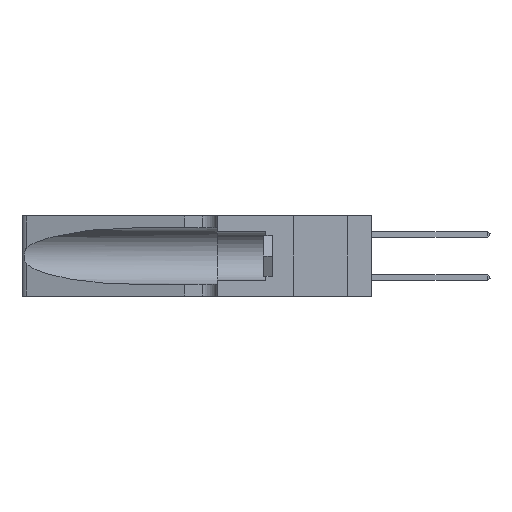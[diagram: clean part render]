
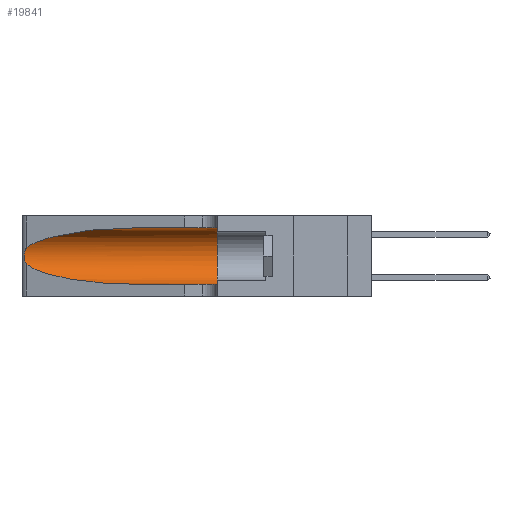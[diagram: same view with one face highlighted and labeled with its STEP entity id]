
A CAD part, left-side view. The second image highlights one B-rep face of the part: STEP entity #19841.
In plain terms, the highlighted cylindrical face has radius 3.308 mm (diameter 6.617 mm), a partial arc.
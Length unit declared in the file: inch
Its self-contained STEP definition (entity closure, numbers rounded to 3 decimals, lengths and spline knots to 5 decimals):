
#235 = CARTESIAN_POINT ( 'NONE',  ( 0.1305, 0.35, 0.185 ) ) ;
#570 = CARTESIAN_POINT ( 'NONE',  ( 0.25639, 1.23186, 0.15144 ) ) ;
#790 = CARTESIAN_POINT ( 'NONE',  ( 0.26017, 1.23833, 0.17102 ) ) ;
#1086 =( BOUNDED_CURVE ( )  B_SPLINE_CURVE ( 3, ( #15805, #12935, #13164, #20333 ),
 .UNSPECIFIED., .F., .F. ) 
 B_SPLINE_CURVE_WITH_KNOTS ( ( 4, 4 ),
 ( 1.5708, 2.84003 ),
 .UNSPECIFIED. ) 
 CURVE ( )  GEOMETRIC_REPRESENTATION_ITEM ( )  RATIONAL_B_SPLINE_CURVE ( ( 1., 0.87, 0.87, 1. ) ) 
 REPRESENTATION_ITEM ( '' )  );
#1731 = DIRECTION ( 'NONE',  ( 0., -1., 0. ) ) ;
#1955 = CARTESIAN_POINT ( 'NONE',  ( 0.1305, 1.61858, 0.31525 ) ) ;
#2019 = CIRCLE ( 'NONE', #22826, 0.13025 ) ;
#2462 = CARTESIAN_POINT ( 'NONE',  ( 0.2373, 1.15595, 0.08982 ) ) ;
#2648 = DIRECTION ( 'NONE',  ( 0., -1., 0. ) ) ;
#2991 = CARTESIAN_POINT ( 'NONE',  ( 0.25487, 1.22718, 0.14631 ) ) ;
#4802 = EDGE_CURVE ( 'NONE', #27854, #12663, #32027, .T. ) ;
#5497 = CARTESIAN_POINT ( 'NONE',  ( 0.25487, 1.22718, 0.22369 ) ) ;
#5634 = CARTESIAN_POINT ( 'NONE',  ( 0.25789, 1.23486, 0.15765 ) ) ;
#5841 = EDGE_CURVE ( 'NONE', #22460, #14654, #16721, .T. ) ;
#6043 = EDGE_CURVE ( 'NONE', #14654, #13248, #11455, .T. ) ;
#7438 = DIRECTION ( 'NONE',  ( 0., 0., 1. ) ) ;
#7979 = CARTESIAN_POINT ( 'NONE',  ( 0.26075, 1.23896, 0.178 ) ) ;
#7989 = ORIENTED_EDGE ( 'NONE', *, *, #20329, .F. ) ;
#8063 = CARTESIAN_POINT ( 'NONE',  ( 0.1305, 1.61858, 0.05475 ) ) ;
#8187 = CARTESIAN_POINT ( 'NONE',  ( 0.26075, 1.23896, 0.19203 ) ) ;
#10887 = CARTESIAN_POINT ( 'NONE',  ( 0.25787, 1.23484, 0.2124 ) ) ;
#11156 = ORIENTED_EDGE ( 'NONE', *, *, #4802, .F. ) ;
#11455 = LINE ( 'NONE', #8063, #18912 ) ;
#12663 = VERTEX_POINT ( 'NONE', #20535 ) ;
#12935 = CARTESIAN_POINT ( 'NONE',  ( 0.18966, 0.96281, 0.31525 ) ) ;
#13164 = CARTESIAN_POINT ( 'NONE',  ( 0.2373, 1.15595, 0.28018 ) ) ;
#13248 = VERTEX_POINT ( 'NONE', #27763 ) ;
#13956 = CYLINDRICAL_SURFACE ( 'NONE', #25717, 0.13025 ) ;
#14654 = VERTEX_POINT ( 'NONE', #27692 ) ;
#14758 = CARTESIAN_POINT ( 'NONE',  ( 0.1305, 0.72297, 0.05475 ) ) ;
#15805 = CARTESIAN_POINT ( 'NONE',  ( 0.1305, 0.72297, 0.31525 ) ) ;
#15926 = FACE_OUTER_BOUND ( 'NONE', #27767, .T. ) ;
#16721 =( BOUNDED_CURVE ( )  B_SPLINE_CURVE ( 3, ( #17593, #2462, #30049, #14758 ),
 .UNSPECIFIED., .F., .F. ) 
 B_SPLINE_CURVE_WITH_KNOTS ( ( 4, 4 ),
 ( 3.44316, 4.71239 ),
 .UNSPECIFIED. ) 
 CURVE ( )  GEOMETRIC_REPRESENTATION_ITEM ( )  RATIONAL_B_SPLINE_CURVE ( ( 1., 0.87, 0.87, 1. ) ) 
 REPRESENTATION_ITEM ( '' )  );
#17593 = CARTESIAN_POINT ( 'NONE',  ( 0.25487, 1.22718, 0.14631 ) ) ;
#17687 = VERTEX_POINT ( 'NONE', #5497 ) ;
#18127 = CARTESIAN_POINT ( 'NONE',  ( 0.25856, 1.23593, 0.16098 ) ) ;
#18912 = VECTOR ( 'NONE', #2648, 39.37008 ) ;
#19402 = DIRECTION ( 'NONE',  ( 0., -1., 0. ) ) ;
#19419 = VECTOR ( 'NONE', #1731, 39.37008 ) ;
#19627 = ORIENTED_EDGE ( 'NONE', *, *, #25099, .T. ) ;
#19841 = ADVANCED_FACE ( 'NONE', ( #15926 ), #13956, .F. ) ;
#20329 = EDGE_CURVE ( 'NONE', #12663, #13248, #2019, .T. ) ;
#20333 = CARTESIAN_POINT ( 'NONE',  ( 0.25487, 1.22718, 0.22369 ) ) ;
#20535 = CARTESIAN_POINT ( 'NONE',  ( 0.1305, 0.35, 0.31525 ) ) ;
#20575 = CARTESIAN_POINT ( 'NONE',  ( 0.25555, 1.22994, 0.2215 ) ) ;
#21088 = ORIENTED_EDGE ( 'NONE', *, *, #25924, .T. ) ;
#21905 = CARTESIAN_POINT ( 'NONE',  ( 0.1305, 1.61858, 0.185 ) ) ;
#22135 = B_SPLINE_CURVE_WITH_KNOTS ( 'NONE', 3,
 ( #23424, #20575, #25475, #10887, #30578, #31000, #8187, #7979, #790, #18127, #5634, #570, #23198, #2991 ),
 .UNSPECIFIED., .F., .F.,
 ( 4, 2, 2, 2, 2, 2, 4 ),
 ( 0., 0.00027, 0.00053, 0.00107, 0.0016, 0.00187, 0.00214 ),
 .UNSPECIFIED. ) ;
#22460 = VERTEX_POINT ( 'NONE', #27746 ) ;
#22564 = CARTESIAN_POINT ( 'NONE',  ( 0.1305, 0.72297, 0.31525 ) ) ;
#22566 = DIRECTION ( 'NONE',  ( 0., 1., 0. ) ) ;
#22826 = AXIS2_PLACEMENT_3D ( 'NONE', #235, #22566, #7438 ) ;
#23198 = CARTESIAN_POINT ( 'NONE',  ( 0.25555, 1.22993, 0.14849 ) ) ;
#23424 = CARTESIAN_POINT ( 'NONE',  ( 0.25487, 1.22718, 0.22369 ) ) ;
#24102 = ORIENTED_EDGE ( 'NONE', *, *, #5841, .T. ) ;
#25099 = EDGE_CURVE ( 'NONE', #27854, #17687, #1086, .T. ) ;
#25475 = CARTESIAN_POINT ( 'NONE',  ( 0.25639, 1.23184, 0.21858 ) ) ;
#25717 = AXIS2_PLACEMENT_3D ( 'NONE', #21905, #19402, #26737 ) ;
#25924 = EDGE_CURVE ( 'NONE', #17687, #22460, #22135, .T. ) ;
#26737 = DIRECTION ( 'NONE',  ( 0., 0., -1. ) ) ;
#27692 = CARTESIAN_POINT ( 'NONE',  ( 0.1305, 0.72297, 0.05475 ) ) ;
#27746 = CARTESIAN_POINT ( 'NONE',  ( 0.25487, 1.22718, 0.14631 ) ) ;
#27763 = CARTESIAN_POINT ( 'NONE',  ( 0.1305, 0.35, 0.05475 ) ) ;
#27767 = EDGE_LOOP ( 'NONE', ( #19627, #21088, #24102, #28614, #7989, #11156 ) ) ;
#27854 = VERTEX_POINT ( 'NONE', #22564 ) ;
#28614 = ORIENTED_EDGE ( 'NONE', *, *, #6043, .T. ) ;
#30049 = CARTESIAN_POINT ( 'NONE',  ( 0.18966, 0.96281, 0.05475 ) ) ;
#30578 = CARTESIAN_POINT ( 'NONE',  ( 0.25854, 1.2359, 0.20912 ) ) ;
#31000 = CARTESIAN_POINT ( 'NONE',  ( 0.26018, 1.23835, 0.19895 ) ) ;
#32027 = LINE ( 'NONE', #1955, #19419 ) ;
